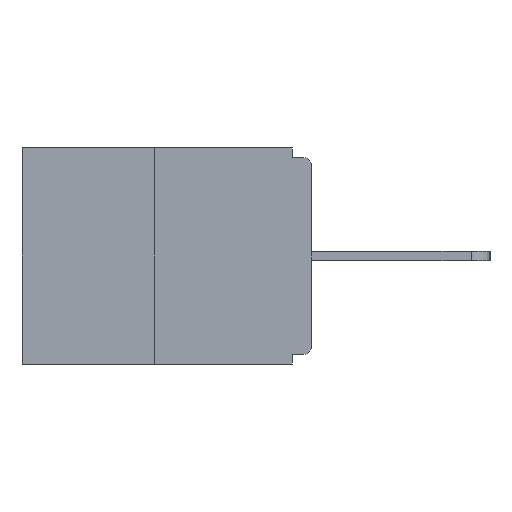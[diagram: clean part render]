
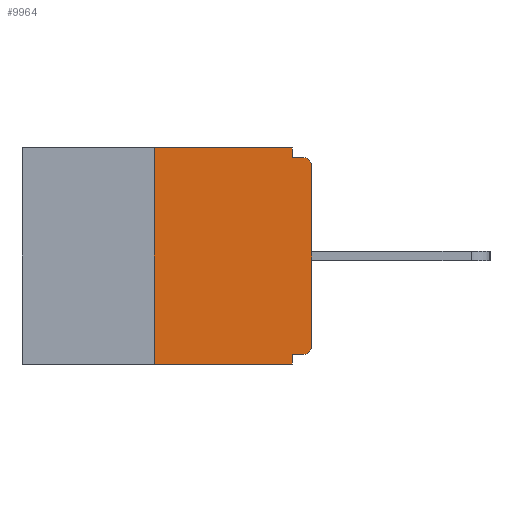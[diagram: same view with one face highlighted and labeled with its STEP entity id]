
A CAD part, left-side view. The second image highlights one B-rep face of the part: STEP entity #9964.
In plain terms, the highlighted planar face has unit normal (-1, 0, 0).
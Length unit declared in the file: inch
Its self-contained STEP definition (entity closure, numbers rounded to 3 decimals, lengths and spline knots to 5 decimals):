
#450 = DIRECTION ( 'NONE',  ( 1., 0., 0. ) ) ;
#463 = VECTOR ( 'NONE', #11599, 39.37008 ) ;
#518 = CARTESIAN_POINT ( 'NONE',  ( 0., 0.031, -0.343 ) ) ;
#564 = PLANE ( 'NONE',  #11479 ) ;
#721 = DIRECTION ( 'NONE',  ( 0., -1., 0. ) ) ;
#814 = CARTESIAN_POINT ( 'NONE',  ( 0., 0.031, -0.328 ) ) ;
#1124 = EDGE_LOOP ( 'NONE', ( #9679, #2030, #6549, #6710, #4249, #11495, #8489, #3232, #3424, #8725 ) ) ;
#1397 = VECTOR ( 'NONE', #3235, 39.37008 ) ;
#1398 = DIRECTION ( 'NONE',  ( 0., 1., 0. ) ) ;
#1909 = CARTESIAN_POINT ( 'NONE',  ( 0., 0., 0. ) ) ;
#1990 = VERTEX_POINT ( 'NONE', #6509 ) ;
#2030 = ORIENTED_EDGE ( 'NONE', *, *, #5065, .F. ) ;
#2348 = EDGE_CURVE ( 'NONE', #5261, #5185, #5795, .T. ) ;
#2395 = DIRECTION ( 'NONE',  ( 0., 0., -1. ) ) ;
#2513 = CARTESIAN_POINT ( 'NONE',  ( 0., 0.46, 0. ) ) ;
#2638 = CARTESIAN_POINT ( 'NONE',  ( 0., 0.015, -0.328 ) ) ;
#2704 = EDGE_CURVE ( 'NONE', #2721, #1990, #5014, .T. ) ;
#2721 = VERTEX_POINT ( 'NONE', #814 ) ;
#2750 = EDGE_CURVE ( 'NONE', #7785, #5185, #8013, .T. ) ;
#3100 = CARTESIAN_POINT ( 'NONE',  ( 0., 0.015, -0.03 ) ) ;
#3140 = CARTESIAN_POINT ( 'NONE',  ( 0., 0.015, -0.015 ) ) ;
#3163 = FACE_OUTER_BOUND ( 'NONE', #1124, .T. ) ;
#3222 = DIRECTION ( 'NONE',  ( 0., 0., -1. ) ) ;
#3232 = ORIENTED_EDGE ( 'NONE', *, *, #2348, .T. ) ;
#3235 = DIRECTION ( 'NONE',  ( 0., 0., -1. ) ) ;
#3424 = ORIENTED_EDGE ( 'NONE', *, *, #2750, .F. ) ;
#3543 = VECTOR ( 'NONE', #8040, 39.37008 ) ;
#3576 = EDGE_CURVE ( 'NONE', #7770, #7785, #9916, .T. ) ;
#3685 = EDGE_CURVE ( 'NONE', #6764, #7770, #9686, .T. ) ;
#3709 = AXIS2_PLACEMENT_3D ( 'NONE', #3100, #4927, #8511 ) ;
#4249 = ORIENTED_EDGE ( 'NONE', *, *, #10485, .F. ) ;
#4344 = VECTOR ( 'NONE', #1398, 39.37008 ) ;
#4787 = VECTOR ( 'NONE', #10916, 39.37008 ) ;
#4908 = EDGE_CURVE ( 'NONE', #9122, #5261, #9976, .T. ) ;
#4927 = DIRECTION ( 'NONE',  ( -1., 0., 0. ) ) ;
#5014 = LINE ( 'NONE', #518, #1397 ) ;
#5065 = EDGE_CURVE ( 'NONE', #5863, #6764, #7578, .T. ) ;
#5185 = VERTEX_POINT ( 'NONE', #3140 ) ;
#5261 = VERTEX_POINT ( 'NONE', #11494 ) ;
#5485 = CARTESIAN_POINT ( 'NONE',  ( 0., 0., -0.015 ) ) ;
#5524 = DIRECTION ( 'NONE',  ( 0., 0., 1. ) ) ;
#5622 = CARTESIAN_POINT ( 'NONE',  ( 0., 0.031, -0.015 ) ) ;
#5656 = VECTOR ( 'NONE', #721, 39.37008 ) ;
#5787 = VERTEX_POINT ( 'NONE', #2638 ) ;
#5795 = CIRCLE ( 'NONE', #3709, 0.015 ) ;
#5863 = VERTEX_POINT ( 'NONE', #10952 ) ;
#5978 = EDGE_CURVE ( 'NONE', #5787, #9122, #9651, .T. ) ;
#6479 = AXIS2_PLACEMENT_3D ( 'NONE', #10287, #8586, #2395 ) ;
#6509 = CARTESIAN_POINT ( 'NONE',  ( 0., 0.031, -0.343 ) ) ;
#6549 = ORIENTED_EDGE ( 'NONE', *, *, #6714, .T. ) ;
#6710 = ORIENTED_EDGE ( 'NONE', *, *, #2704, .F. ) ;
#6714 = EDGE_CURVE ( 'NONE', #5863, #1990, #8939, .T. ) ;
#6764 = VERTEX_POINT ( 'NONE', #10060 ) ;
#6789 = VECTOR ( 'NONE', #8717, 39.37008 ) ;
#6846 = CARTESIAN_POINT ( 'NONE',  ( 0., 0., -0.328 ) ) ;
#7097 = CARTESIAN_POINT ( 'NONE',  ( 0., 0., -0.313 ) ) ;
#7504 = CARTESIAN_POINT ( 'NONE',  ( 0., 0.031, 0. ) ) ;
#7578 = LINE ( 'NONE', #8337, #4787 ) ;
#7770 = VERTEX_POINT ( 'NONE', #7504 ) ;
#7785 = VERTEX_POINT ( 'NONE', #5622 ) ;
#8013 = LINE ( 'NONE', #5485, #463 ) ;
#8040 = DIRECTION ( 'NONE',  ( 0., 0., -1. ) ) ;
#8337 = CARTESIAN_POINT ( 'NONE',  ( 0., 0.25, 0. ) ) ;
#8489 = ORIENTED_EDGE ( 'NONE', *, *, #4908, .T. ) ;
#8511 = DIRECTION ( 'NONE',  ( 0., 0., -1. ) ) ;
#8586 = DIRECTION ( 'NONE',  ( -1., 0., 0. ) ) ;
#8717 = DIRECTION ( 'NONE',  ( 0., -1., 0. ) ) ;
#8725 = ORIENTED_EDGE ( 'NONE', *, *, #3576, .F. ) ;
#8804 = CARTESIAN_POINT ( 'NONE',  ( 0., 0.46, 0. ) ) ;
#8939 = LINE ( 'NONE', #11535, #6789 ) ;
#9122 = VERTEX_POINT ( 'NONE', #7097 ) ;
#9333 = VECTOR ( 'NONE', #5524, 39.37008 ) ;
#9488 = LINE ( 'NONE', #6846, #4344 ) ;
#9651 = CIRCLE ( 'NONE', #6479, 0.015 ) ;
#9679 = ORIENTED_EDGE ( 'NONE', *, *, #3685, .F. ) ;
#9686 = LINE ( 'NONE', #8804, #5656 ) ;
#9804 = CARTESIAN_POINT ( 'NONE',  ( 0., 0.031, 0. ) ) ;
#9916 = LINE ( 'NONE', #9804, #3543 ) ;
#9964 = ADVANCED_FACE ( 'NONE', ( #3163 ), #564, .F. ) ;
#9976 = LINE ( 'NONE', #1909, #9333 ) ;
#10060 = CARTESIAN_POINT ( 'NONE',  ( 0., 0.25, 0. ) ) ;
#10287 = CARTESIAN_POINT ( 'NONE',  ( 0., 0.015, -0.313 ) ) ;
#10485 = EDGE_CURVE ( 'NONE', #5787, #2721, #9488, .T. ) ;
#10916 = DIRECTION ( 'NONE',  ( 0., 0., 1. ) ) ;
#10952 = CARTESIAN_POINT ( 'NONE',  ( 0., 0.25, -0.343 ) ) ;
#11479 = AXIS2_PLACEMENT_3D ( 'NONE', #2513, #450, #3222 ) ;
#11494 = CARTESIAN_POINT ( 'NONE',  ( 0., 0., -0.03 ) ) ;
#11495 = ORIENTED_EDGE ( 'NONE', *, *, #5978, .T. ) ;
#11535 = CARTESIAN_POINT ( 'NONE',  ( 0., 0.46, -0.343 ) ) ;
#11599 = DIRECTION ( 'NONE',  ( 0., -1., 0. ) ) ;
